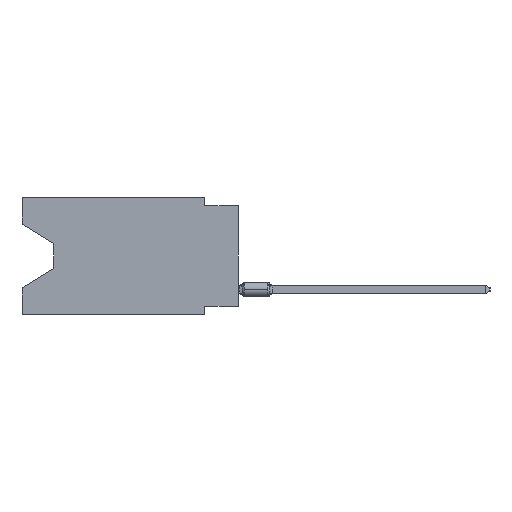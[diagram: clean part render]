
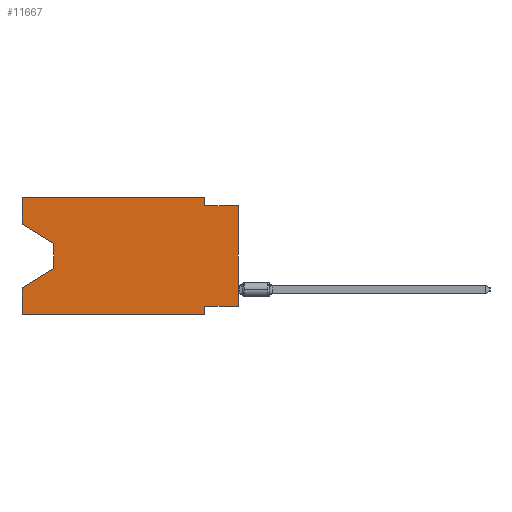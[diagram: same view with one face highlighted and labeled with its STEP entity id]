
A CAD part, left-side view. The second image highlights one B-rep face of the part: STEP entity #11667.
In plain terms, the highlighted planar face has unit normal (-1, 0, 0).
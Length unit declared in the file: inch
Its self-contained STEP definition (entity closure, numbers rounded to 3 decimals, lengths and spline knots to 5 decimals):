
#77 = VECTOR ( 'NONE', #14649, 39.37008 ) ;
#146 = VERTEX_POINT ( 'NONE', #14981 ) ;
#249 = DIRECTION ( 'NONE',  ( 0., -0.855, -0.519 ) ) ;
#802 = DIRECTION ( 'NONE',  ( 0., -1., 0. ) ) ;
#1092 = CARTESIAN_POINT ( 'NONE',  ( 0., 0.645, -0.08025 ) ) ;
#1181 = VECTOR ( 'NONE', #249, 39.37008 ) ;
#1214 = DIRECTION ( 'NONE',  ( 0., 0., 1. ) ) ;
#1689 = ORIENTED_EDGE ( 'NONE', *, *, #3476, .T. ) ;
#1788 = VECTOR ( 'NONE', #15694, 39.37008 ) ;
#1961 = CARTESIAN_POINT ( 'NONE',  ( 0., 0.1, -0.325 ) ) ;
#2043 = ORIENTED_EDGE ( 'NONE', *, *, #17060, .T. ) ;
#2222 = ORIENTED_EDGE ( 'NONE', *, *, #16434, .F. ) ;
#2394 = VERTEX_POINT ( 'NONE', #1092 ) ;
#2595 = ORIENTED_EDGE ( 'NONE', *, *, #3932, .F. ) ;
#3239 = CARTESIAN_POINT ( 'NONE',  ( 0., 0.1, 0. ) ) ;
#3376 = DIRECTION ( 'NONE',  ( 0., 0., -1. ) ) ;
#3430 = CARTESIAN_POINT ( 'NONE',  ( 0., 0., -0.325 ) ) ;
#3476 = EDGE_CURVE ( 'NONE', #14440, #12244, #4506, .T. ) ;
#3685 = CARTESIAN_POINT ( 'NONE',  ( 0., 0.55, -0.138 ) ) ;
#3932 = EDGE_CURVE ( 'NONE', #4265, #9382, #6039, .T. ) ;
#3977 = DIRECTION ( 'NONE',  ( 0., 0., 1. ) ) ;
#4223 = VERTEX_POINT ( 'NONE', #3239 ) ;
#4265 = VERTEX_POINT ( 'NONE', #1961 ) ;
#4506 = LINE ( 'NONE', #10105, #1788 ) ;
#4514 = DIRECTION ( 'NONE',  ( 0., 0., -1. ) ) ;
#4853 = CARTESIAN_POINT ( 'NONE',  ( 0., 0.1, -0.025 ) ) ;
#4951 = VECTOR ( 'NONE', #1214, 39.37008 ) ;
#5035 = VECTOR ( 'NONE', #3376, 39.37008 ) ;
#5103 = VECTOR ( 'NONE', #14615, 39.37008 ) ;
#5108 = ORIENTED_EDGE ( 'NONE', *, *, #11773, .F. ) ;
#5129 = VERTEX_POINT ( 'NONE', #4853 ) ;
#5149 = EDGE_LOOP ( 'NONE', ( #10829, #2043, #1689, #7706, #12873, #2595, #18003, #16966, #16342, #5108, #9241, #2222 ) ) ;
#5293 = LINE ( 'NONE', #7767, #14746 ) ;
#5390 = EDGE_CURVE ( 'NONE', #13840, #4223, #10987, .T. ) ;
#5894 = DIRECTION ( 'NONE',  ( 0., 0., -1. ) ) ;
#5982 = CARTESIAN_POINT ( 'NONE',  ( 0., 0.1, 0. ) ) ;
#6039 = LINE ( 'NONE', #10622, #5035 ) ;
#6267 = EDGE_CURVE ( 'NONE', #5129, #10603, #11277, .T. ) ;
#6361 = AXIS2_PLACEMENT_3D ( 'NONE', #11481, #10378, #5894 ) ;
#6517 = CARTESIAN_POINT ( 'NONE',  ( 0., 0., -0.025 ) ) ;
#7267 = LINE ( 'NONE', #8738, #15452 ) ;
#7444 = FACE_OUTER_BOUND ( 'NONE', #5149, .T. ) ;
#7706 = ORIENTED_EDGE ( 'NONE', *, *, #15291, .F. ) ;
#7767 = CARTESIAN_POINT ( 'NONE',  ( 0., 0.645, -0.35 ) ) ;
#8002 = EDGE_CURVE ( 'NONE', #16914, #9382, #5293, .T. ) ;
#8367 = EDGE_CURVE ( 'NONE', #146, #4265, #16001, .T. ) ;
#8452 = CARTESIAN_POINT ( 'NONE',  ( 0., 0.645, 0. ) ) ;
#8497 = DIRECTION ( 'NONE',  ( 0., 0., -1. ) ) ;
#8503 = VECTOR ( 'NONE', #8497, 39.37008 ) ;
#8738 = CARTESIAN_POINT ( 'NONE',  ( 0., 0., 0. ) ) ;
#9068 = CARTESIAN_POINT ( 'NONE',  ( 0., 0.1, -0.35 ) ) ;
#9241 = ORIENTED_EDGE ( 'NONE', *, *, #5390, .F. ) ;
#9382 = VERTEX_POINT ( 'NONE', #9068 ) ;
#10105 = CARTESIAN_POINT ( 'NONE',  ( 0., 0.55, -0.212 ) ) ;
#10117 = CARTESIAN_POINT ( 'NONE',  ( 0., 0.645, 0. ) ) ;
#10146 = LINE ( 'NONE', #12711, #1181 ) ;
#10288 = PLANE ( 'NONE',  #6361 ) ;
#10378 = DIRECTION ( 'NONE',  ( 1., 0., 0. ) ) ;
#10603 = VERTEX_POINT ( 'NONE', #6517 ) ;
#10622 = CARTESIAN_POINT ( 'NONE',  ( 0., 0.1, -0.35 ) ) ;
#10829 = ORIENTED_EDGE ( 'NONE', *, *, #16338, .T. ) ;
#10987 = LINE ( 'NONE', #16679, #14148 ) ;
#11037 = LINE ( 'NONE', #16543, #14632 ) ;
#11277 = LINE ( 'NONE', #15498, #77 ) ;
#11481 = CARTESIAN_POINT ( 'NONE',  ( 0., 0.645, 0. ) ) ;
#11514 = CARTESIAN_POINT ( 'NONE',  ( 0., 0.55, -0.212 ) ) ;
#11667 = ADVANCED_FACE ( 'NONE', ( #7444 ), #10288, .F. ) ;
#11773 = EDGE_CURVE ( 'NONE', #4223, #5129, #14495, .T. ) ;
#12244 = VERTEX_POINT ( 'NONE', #17507 ) ;
#12477 = LINE ( 'NONE', #8452, #4951 ) ;
#12711 = CARTESIAN_POINT ( 'NONE',  ( 0., 0.645, -0.08025 ) ) ;
#12873 = ORIENTED_EDGE ( 'NONE', *, *, #8002, .T. ) ;
#13027 = DIRECTION ( 'NONE',  ( 0., 0., 1. ) ) ;
#13379 = VECTOR ( 'NONE', #4514, 39.37008 ) ;
#13470 = CARTESIAN_POINT ( 'NONE',  ( 0., 0.645, -0.35 ) ) ;
#13776 = EDGE_CURVE ( 'NONE', #146, #10603, #7267, .T. ) ;
#13840 = VERTEX_POINT ( 'NONE', #10117 ) ;
#14148 = VECTOR ( 'NONE', #18142, 39.37008 ) ;
#14260 = LINE ( 'NONE', #17209, #8503 ) ;
#14440 = VERTEX_POINT ( 'NONE', #11514 ) ;
#14495 = LINE ( 'NONE', #5982, #13379 ) ;
#14615 = DIRECTION ( 'NONE',  ( 0., 1., 0. ) ) ;
#14632 = VECTOR ( 'NONE', #3977, 39.37008 ) ;
#14649 = DIRECTION ( 'NONE',  ( 0., -1., 0. ) ) ;
#14746 = VECTOR ( 'NONE', #802, 39.37008 ) ;
#14981 = CARTESIAN_POINT ( 'NONE',  ( 0., 0., -0.325 ) ) ;
#15083 = VERTEX_POINT ( 'NONE', #3685 ) ;
#15291 = EDGE_CURVE ( 'NONE', #16914, #12244, #12477, .T. ) ;
#15452 = VECTOR ( 'NONE', #13027, 39.37008 ) ;
#15498 = CARTESIAN_POINT ( 'NONE',  ( 0., 0., -0.025 ) ) ;
#15694 = DIRECTION ( 'NONE',  ( 0., 0.855, -0.519 ) ) ;
#16001 = LINE ( 'NONE', #3430, #5103 ) ;
#16338 = EDGE_CURVE ( 'NONE', #2394, #15083, #10146, .T. ) ;
#16342 = ORIENTED_EDGE ( 'NONE', *, *, #6267, .F. ) ;
#16434 = EDGE_CURVE ( 'NONE', #2394, #13840, #11037, .T. ) ;
#16543 = CARTESIAN_POINT ( 'NONE',  ( 0., 0.645, 0. ) ) ;
#16679 = CARTESIAN_POINT ( 'NONE',  ( 0., 0.645, 0. ) ) ;
#16914 = VERTEX_POINT ( 'NONE', #13470 ) ;
#16966 = ORIENTED_EDGE ( 'NONE', *, *, #13776, .T. ) ;
#17060 = EDGE_CURVE ( 'NONE', #15083, #14440, #14260, .T. ) ;
#17209 = CARTESIAN_POINT ( 'NONE',  ( 0., 0.55, -0.138 ) ) ;
#17507 = CARTESIAN_POINT ( 'NONE',  ( 0., 0.645, -0.26975 ) ) ;
#18003 = ORIENTED_EDGE ( 'NONE', *, *, #8367, .F. ) ;
#18142 = DIRECTION ( 'NONE',  ( 0., -1., 0. ) ) ;
